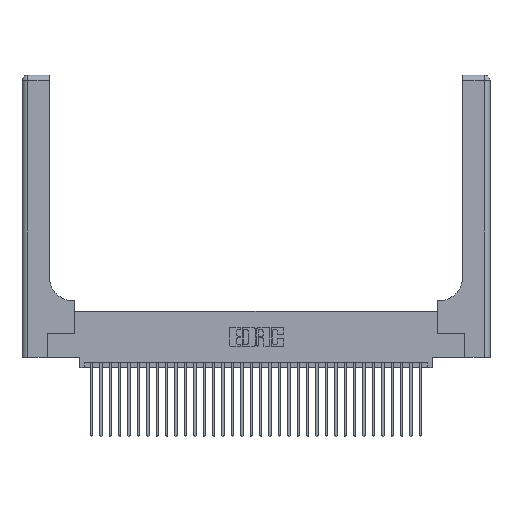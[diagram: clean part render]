
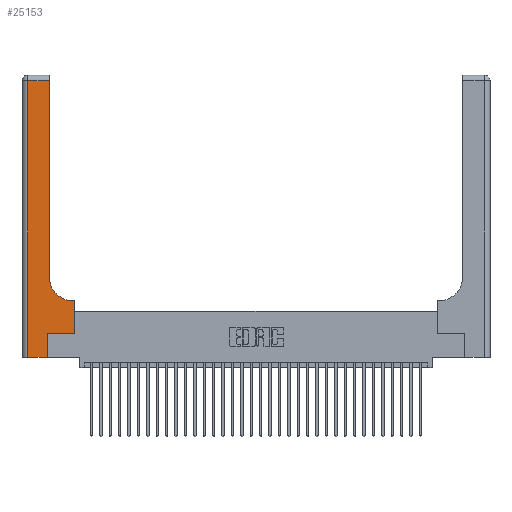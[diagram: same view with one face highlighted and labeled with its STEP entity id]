
A CAD part, top view. The second image highlights one B-rep face of the part: STEP entity #25153.
In plain terms, the highlighted planar face has unit normal (0, 0, 1).
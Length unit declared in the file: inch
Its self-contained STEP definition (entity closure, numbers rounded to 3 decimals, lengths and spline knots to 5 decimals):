
#260 = VERTEX_POINT ( 'NONE', #31790 ) ;
#429 = DIRECTION ( 'NONE',  ( -1., 0., 0. ) ) ;
#492 = CARTESIAN_POINT ( 'NONE',  ( 0.269, 0., 0.37 ) ) ;
#1013 = DIRECTION ( 'NONE',  ( -1., 0., 0. ) ) ;
#1025 = CARTESIAN_POINT ( 'NONE',  ( 0.06, 0., 0.37 ) ) ;
#1083 = DIRECTION ( 'NONE',  ( 1., 0., 0. ) ) ;
#1403 = VERTEX_POINT ( 'NONE', #2210 ) ;
#2210 = CARTESIAN_POINT ( 'NONE',  ( 0.269, 0.25, 0.37 ) ) ;
#2592 = LINE ( 'NONE', #6461, #11253 ) ;
#2987 = CARTESIAN_POINT ( 'NONE',  ( 0.269, 0.25, 0.37 ) ) ;
#4718 = CARTESIAN_POINT ( 'NONE',  ( 0.5585, 0.25, 0.37 ) ) ;
#5039 = LINE ( 'NONE', #10988, #17998 ) ;
#5118 = EDGE_CURVE ( 'NONE', #6893, #1403, #26978, .T. ) ;
#5443 = LINE ( 'NONE', #27426, #17117 ) ;
#6055 = DIRECTION ( 'NONE',  ( 0., -1., 0. ) ) ;
#6194 = AXIS2_PLACEMENT_3D ( 'NONE', #19547, #30228, #1083 ) ;
#6435 = DIRECTION ( 'NONE',  ( 0., 0., -1. ) ) ;
#6461 = CARTESIAN_POINT ( 'NONE',  ( 0.2915, 0.6, 0.37 ) ) ;
#6545 = CARTESIAN_POINT ( 'NONE',  ( 0.5585, 0.25, 0.37 ) ) ;
#6893 = VERTEX_POINT ( 'NONE', #33400 ) ;
#7150 = LINE ( 'NONE', #18091, #27475 ) ;
#7421 = ORIENTED_EDGE ( 'NONE', *, *, #13640, .T. ) ;
#8181 = EDGE_CURVE ( 'NONE', #19916, #28660, #5443, .T. ) ;
#8244 = ORIENTED_EDGE ( 'NONE', *, *, #25970, .T. ) ;
#8877 = PLANE ( 'NONE',  #28338 ) ;
#9126 = VERTEX_POINT ( 'NONE', #10953 ) ;
#10356 = LINE ( 'NONE', #2987, #32362 ) ;
#10435 = EDGE_LOOP ( 'NONE', ( #8244, #15552, #13626, #7421, #11773, #22539, #23012, #23189, #31992 ) ) ;
#10953 = CARTESIAN_POINT ( 'NONE',  ( 0.2915, 2.94, 0.37 ) ) ;
#10988 = CARTESIAN_POINT ( 'NONE',  ( 0., 2.94, 0.37 ) ) ;
#11253 = VECTOR ( 'NONE', #30293, 39.37008 ) ;
#11276 = CIRCLE ( 'NONE', #6194, 0.25 ) ;
#11773 = ORIENTED_EDGE ( 'NONE', *, *, #5118, .T. ) ;
#11849 = VECTOR ( 'NONE', #12734, 39.37008 ) ;
#12734 = DIRECTION ( 'NONE',  ( 0., 1., 0. ) ) ;
#12749 = VERTEX_POINT ( 'NONE', #6545 ) ;
#13626 = ORIENTED_EDGE ( 'NONE', *, *, #8181, .T. ) ;
#13640 = EDGE_CURVE ( 'NONE', #28660, #6893, #32736, .T. ) ;
#14153 = VERTEX_POINT ( 'NONE', #26455 ) ;
#14542 = VECTOR ( 'NONE', #21840, 39.37008 ) ;
#15552 = ORIENTED_EDGE ( 'NONE', *, *, #24526, .T. ) ;
#15772 = DIRECTION ( 'NONE',  ( 1., 0., 0. ) ) ;
#17076 = CARTESIAN_POINT ( 'NONE',  ( 0.06, 2.94, 0.37 ) ) ;
#17117 = VECTOR ( 'NONE', #6055, 39.37008 ) ;
#17276 = EDGE_CURVE ( 'NONE', #14153, #260, #11276, .T. ) ;
#17800 = VERTEX_POINT ( 'NONE', #18898 ) ;
#17998 = VECTOR ( 'NONE', #429, 39.37008 ) ;
#18091 = CARTESIAN_POINT ( 'NONE',  ( 0.2915, 3., 0.37 ) ) ;
#18898 = CARTESIAN_POINT ( 'NONE',  ( 0.5585, 0.6, 0.37 ) ) ;
#19547 = CARTESIAN_POINT ( 'NONE',  ( 0.5415, 0.85, 0.37 ) ) ;
#19749 = EDGE_CURVE ( 'NONE', #1403, #12749, #10356, .T. ) ;
#19916 = VERTEX_POINT ( 'NONE', #17076 ) ;
#20393 = DIRECTION ( 'NONE',  ( 1., 0., 0. ) ) ;
#21840 = DIRECTION ( 'NONE',  ( 0., 1., 0. ) ) ;
#22076 = EDGE_CURVE ( 'NONE', #12749, #17800, #29349, .T. ) ;
#22539 = ORIENTED_EDGE ( 'NONE', *, *, #19749, .T. ) ;
#23012 = ORIENTED_EDGE ( 'NONE', *, *, #22076, .T. ) ;
#23189 = ORIENTED_EDGE ( 'NONE', *, *, #33243, .T. ) ;
#24526 = EDGE_CURVE ( 'NONE', #9126, #19916, #5039, .T. ) ;
#25153 = ADVANCED_FACE ( 'NONE', ( #33297 ), #8877, .F. ) ;
#25834 = DIRECTION ( 'NONE',  ( 0., 1., 0. ) ) ;
#25970 = EDGE_CURVE ( 'NONE', #260, #9126, #7150, .T. ) ;
#26455 = CARTESIAN_POINT ( 'NONE',  ( 0.5415, 0.6, 0.37 ) ) ;
#26978 = LINE ( 'NONE', #492, #14542 ) ;
#27426 = CARTESIAN_POINT ( 'NONE',  ( 0.06, 3., 0.37 ) ) ;
#27457 = CARTESIAN_POINT ( 'NONE',  ( 0., 3., 0.37 ) ) ;
#27475 = VECTOR ( 'NONE', #25834, 39.37008 ) ;
#27743 = VECTOR ( 'NONE', #20393, 39.37008 ) ;
#28338 = AXIS2_PLACEMENT_3D ( 'NONE', #27457, #6435, #1013 ) ;
#28660 = VERTEX_POINT ( 'NONE', #1025 ) ;
#29349 = LINE ( 'NONE', #4718, #11849 ) ;
#30228 = DIRECTION ( 'NONE',  ( 0., 0., -1. ) ) ;
#30293 = DIRECTION ( 'NONE',  ( -1., 0., 0. ) ) ;
#31790 = CARTESIAN_POINT ( 'NONE',  ( 0.2915, 0.85, 0.37 ) ) ;
#31992 = ORIENTED_EDGE ( 'NONE', *, *, #17276, .T. ) ;
#32362 = VECTOR ( 'NONE', #15772, 39.37008 ) ;
#32736 = LINE ( 'NONE', #33291, #27743 ) ;
#33243 = EDGE_CURVE ( 'NONE', #17800, #14153, #2592, .T. ) ;
#33291 = CARTESIAN_POINT ( 'NONE',  ( 0., 0., 0.37 ) ) ;
#33297 = FACE_OUTER_BOUND ( 'NONE', #10435, .T. ) ;
#33400 = CARTESIAN_POINT ( 'NONE',  ( 0.269, 0., 0.37 ) ) ;
